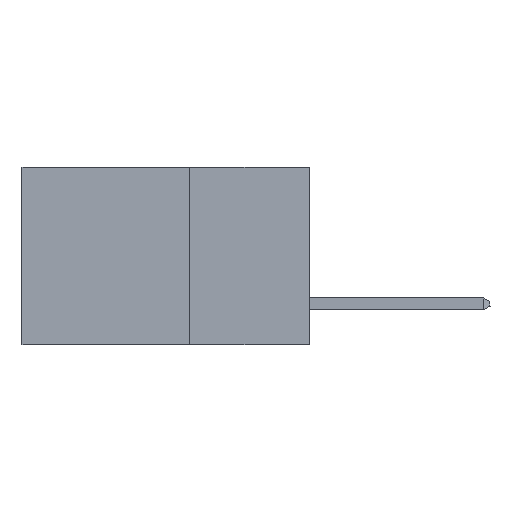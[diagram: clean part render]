
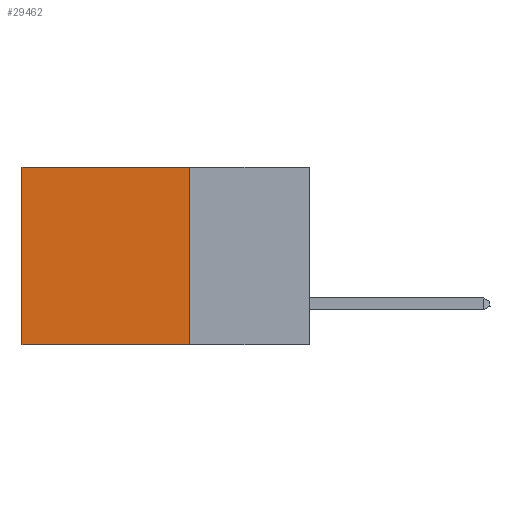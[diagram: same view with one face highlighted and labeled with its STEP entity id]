
A CAD part, left-side view. The second image highlights one B-rep face of the part: STEP entity #29462.
In plain terms, the highlighted planar face has unit normal (-1, 0, 0).
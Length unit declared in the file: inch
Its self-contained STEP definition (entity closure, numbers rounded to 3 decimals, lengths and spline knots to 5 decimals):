
#2101 = VECTOR ( 'NONE', #27248, 39.37008 ) ;
#2552 = DIRECTION ( 'NONE',  ( 0., 0., -1. ) ) ;
#3258 = CARTESIAN_POINT ( 'NONE',  ( 0.2875, 0.25, -0.37 ) ) ;
#4068 = CARTESIAN_POINT ( 'NONE',  ( 0.2875, 0.6, 0. ) ) ;
#4441 = CARTESIAN_POINT ( 'NONE',  ( 0.2875, 0.25, 0. ) ) ;
#5040 = VERTEX_POINT ( 'NONE', #4068 ) ;
#6022 = AXIS2_PLACEMENT_3D ( 'NONE', #4441, #7145, #24995 ) ;
#6689 = VECTOR ( 'NONE', #27359, 39.37008 ) ;
#7145 = DIRECTION ( 'NONE',  ( 1., 0., 0. ) ) ;
#7716 = EDGE_CURVE ( 'NONE', #5040, #16325, #32403, .T. ) ;
#9831 = FACE_OUTER_BOUND ( 'NONE', #26898, .T. ) ;
#10799 = LINE ( 'NONE', #22951, #13400 ) ;
#11237 = EDGE_CURVE ( 'NONE', #14776, #16325, #28971, .T. ) ;
#13400 = VECTOR ( 'NONE', #2552, 39.37008 ) ;
#14776 = VERTEX_POINT ( 'NONE', #3258 ) ;
#14983 = EDGE_CURVE ( 'NONE', #32009, #14776, #10799, .T. ) ;
#15847 = DIRECTION ( 'NONE',  ( 0., 1., 0. ) ) ;
#16285 = ORIENTED_EDGE ( 'NONE', *, *, #11237, .F. ) ;
#16325 = VERTEX_POINT ( 'NONE', #26798 ) ;
#16972 = CARTESIAN_POINT ( 'NONE',  ( 0.2875, 0.25, 0. ) ) ;
#17094 = PLANE ( 'NONE',  #6022 ) ;
#21921 = VECTOR ( 'NONE', #15847, 39.37008 ) ;
#21936 = ORIENTED_EDGE ( 'NONE', *, *, #14983, .F. ) ;
#22034 = LINE ( 'NONE', #16972, #2101 ) ;
#22951 = CARTESIAN_POINT ( 'NONE',  ( 0.2875, 0.25, 0. ) ) ;
#24995 = DIRECTION ( 'NONE',  ( 0., 0., -1. ) ) ;
#26120 = ORIENTED_EDGE ( 'NONE', *, *, #28815, .T. ) ;
#26798 = CARTESIAN_POINT ( 'NONE',  ( 0.2875, 0.6, -0.37 ) ) ;
#26898 = EDGE_LOOP ( 'NONE', ( #30410, #16285, #21936, #26120 ) ) ;
#27028 = CARTESIAN_POINT ( 'NONE',  ( 0.2875, 0.6, 0. ) ) ;
#27248 = DIRECTION ( 'NONE',  ( 0., 1., 0. ) ) ;
#27359 = DIRECTION ( 'NONE',  ( 0., 0., -1. ) ) ;
#28642 = CARTESIAN_POINT ( 'NONE',  ( 0.2875, 0.25, -0.37 ) ) ;
#28815 = EDGE_CURVE ( 'NONE', #32009, #5040, #22034, .T. ) ;
#28971 = LINE ( 'NONE', #28642, #21921 ) ;
#29462 = ADVANCED_FACE ( 'NONE', ( #9831 ), #17094, .F. ) ;
#30410 = ORIENTED_EDGE ( 'NONE', *, *, #7716, .T. ) ;
#32009 = VERTEX_POINT ( 'NONE', #32637 ) ;
#32403 = LINE ( 'NONE', #27028, #6689 ) ;
#32637 = CARTESIAN_POINT ( 'NONE',  ( 0.2875, 0.25, 0. ) ) ;
